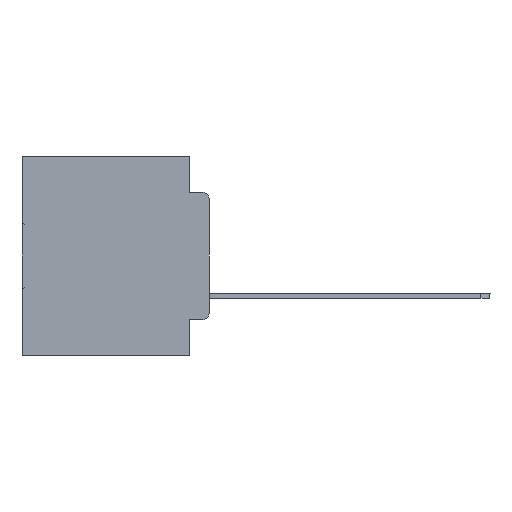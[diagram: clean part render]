
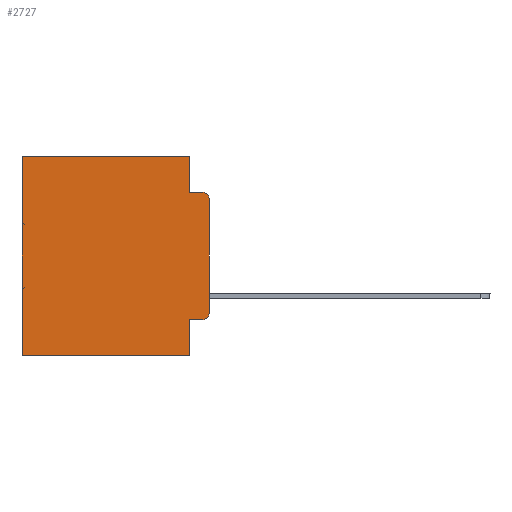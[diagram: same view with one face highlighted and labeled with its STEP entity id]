
A CAD part, left-side view. The second image highlights one B-rep face of the part: STEP entity #2727.
In plain terms, the highlighted planar face has unit normal (-1, 0, 0).
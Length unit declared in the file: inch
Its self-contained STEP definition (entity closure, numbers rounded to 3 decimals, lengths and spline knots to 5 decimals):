
#1617 = DIRECTION ( 'NONE',  ( 0., -1., 0. ) ) ;
#2645 = LINE ( 'NONE', #10070, #27290 ) ;
#2679 = ORIENTED_EDGE ( 'NONE', *, *, #4344, .F. ) ;
#2701 = ORIENTED_EDGE ( 'NONE', *, *, #13896, .F. ) ;
#2727 = ADVANCED_FACE ( 'NONE', ( #23190 ), #23687, .F. ) ;
#3690 = CARTESIAN_POINT ( 'NONE',  ( 0.298, 0.02, -0.4115 ) ) ;
#4344 = EDGE_CURVE ( 'NONE', #23893, #30418, #20851, .T. ) ;
#5278 = VERTEX_POINT ( 'NONE', #13805 ) ;
#5730 = DIRECTION ( 'NONE',  ( 0., 0., -1. ) ) ;
#6343 = ORIENTED_EDGE ( 'NONE', *, *, #31186, .F. ) ;
#6917 = LINE ( 'NONE', #28283, #15752 ) ;
#7305 = DIRECTION ( 'NONE',  ( 0., 0., -1. ) ) ;
#7715 = DIRECTION ( 'NONE',  ( 0., 0., -1. ) ) ;
#8088 = CARTESIAN_POINT ( 'NONE',  ( 0.298, 0.051, 0. ) ) ;
#8089 = DIRECTION ( 'NONE',  ( 1., 0., 0. ) ) ;
#8579 = CARTESIAN_POINT ( 'NONE',  ( 0.298, 0., -0.5 ) ) ;
#9032 = VERTEX_POINT ( 'NONE', #23103 ) ;
#9220 = VERTEX_POINT ( 'NONE', #29182 ) ;
#9267 = ORIENTED_EDGE ( 'NONE', *, *, #15329, .T. ) ;
#9557 = VERTEX_POINT ( 'NONE', #3690 ) ;
#9857 = EDGE_CURVE ( 'NONE', #23893, #5278, #28074, .T. ) ;
#10055 = LINE ( 'NONE', #28208, #25233 ) ;
#10070 = CARTESIAN_POINT ( 'NONE',  ( 0.298, 0., 0. ) ) ;
#11087 = CARTESIAN_POINT ( 'NONE',  ( 0.298, 0.473, -0.5 ) ) ;
#11134 = VECTOR ( 'NONE', #24522, 39.37008 ) ;
#11430 = AXIS2_PLACEMENT_3D ( 'NONE', #30977, #8089, #5730 ) ;
#11694 = ORIENTED_EDGE ( 'NONE', *, *, #18281, .T. ) ;
#12052 = DIRECTION ( 'NONE',  ( 0., 0., -1. ) ) ;
#12464 = CARTESIAN_POINT ( 'NONE',  ( 0.298, 0.02, -0.1085 ) ) ;
#12587 = VERTEX_POINT ( 'NONE', #25571 ) ;
#12720 = DIRECTION ( 'NONE',  ( 0., 0., -1. ) ) ;
#12936 = DIRECTION ( 'NONE',  ( 0., -1., 0. ) ) ;
#12950 = DIRECTION ( 'NONE',  ( 0., 1., 0. ) ) ;
#13708 = VECTOR ( 'NONE', #12720, 39.37008 ) ;
#13805 = CARTESIAN_POINT ( 'NONE',  ( 0.298, 0.02, -0.0885 ) ) ;
#13896 = EDGE_CURVE ( 'NONE', #14059, #12587, #6917, .T. ) ;
#13926 = CARTESIAN_POINT ( 'NONE',  ( 0.298, 0.051, 0. ) ) ;
#14059 = VERTEX_POINT ( 'NONE', #8088 ) ;
#14183 = CIRCLE ( 'NONE', #32062, 0.02 ) ;
#15329 = EDGE_CURVE ( 'NONE', #9557, #30418, #14183, .T. ) ;
#15752 = VECTOR ( 'NONE', #19982, 39.37008 ) ;
#16455 = VECTOR ( 'NONE', #1617, 39.37008 ) ;
#17025 = LINE ( 'NONE', #19911, #16455 ) ;
#17555 = DIRECTION ( 'NONE',  ( -1., 0., 0. ) ) ;
#18143 = DIRECTION ( 'NONE',  ( -1., 0., 0. ) ) ;
#18281 = EDGE_CURVE ( 'NONE', #14059, #23511, #2645, .T. ) ;
#19208 = EDGE_LOOP ( 'NONE', ( #2679, #32222, #6343, #2701, #11694, #20461, #23949, #25158, #27980, #9267 ) ) ;
#19210 = DIRECTION ( 'NONE',  ( 0., 0., -1. ) ) ;
#19722 = CARTESIAN_POINT ( 'NONE',  ( 0.298, 0.473, 0. ) ) ;
#19911 = CARTESIAN_POINT ( 'NONE',  ( 0.298, 0.051, -0.4115 ) ) ;
#19953 = VERTEX_POINT ( 'NONE', #11087 ) ;
#19982 = DIRECTION ( 'NONE',  ( 0., 0., -1. ) ) ;
#20213 = EDGE_CURVE ( 'NONE', #23511, #19953, #24472, .T. ) ;
#20461 = ORIENTED_EDGE ( 'NONE', *, *, #20213, .T. ) ;
#20851 = LINE ( 'NONE', #26293, #13708 ) ;
#23061 = VECTOR ( 'NONE', #19210, 39.37008 ) ;
#23103 = CARTESIAN_POINT ( 'NONE',  ( 0.298, 0.051, -0.5 ) ) ;
#23188 = EDGE_CURVE ( 'NONE', #9220, #9032, #24946, .T. ) ;
#23190 = FACE_OUTER_BOUND ( 'NONE', #19208, .T. ) ;
#23511 = VERTEX_POINT ( 'NONE', #25464 ) ;
#23687 = PLANE ( 'NONE',  #11430 ) ;
#23893 = VERTEX_POINT ( 'NONE', #24403 ) ;
#23949 = ORIENTED_EDGE ( 'NONE', *, *, #30480, .F. ) ;
#24018 = LINE ( 'NONE', #8579, #11134 ) ;
#24403 = CARTESIAN_POINT ( 'NONE',  ( 0.298, 0., -0.1085 ) ) ;
#24472 = LINE ( 'NONE', #19722, #23061 ) ;
#24522 = DIRECTION ( 'NONE',  ( 0., 1., 0. ) ) ;
#24946 = LINE ( 'NONE', #13926, #28575 ) ;
#25158 = ORIENTED_EDGE ( 'NONE', *, *, #23188, .F. ) ;
#25233 = VECTOR ( 'NONE', #12936, 39.37008 ) ;
#25464 = CARTESIAN_POINT ( 'NONE',  ( 0.298, 0.473, 0. ) ) ;
#25571 = CARTESIAN_POINT ( 'NONE',  ( 0.298, 0.051, -0.0885 ) ) ;
#26293 = CARTESIAN_POINT ( 'NONE',  ( 0.298, 0., 0. ) ) ;
#27290 = VECTOR ( 'NONE', #12950, 39.37008 ) ;
#27345 = EDGE_CURVE ( 'NONE', #9220, #9557, #17025, .T. ) ;
#27980 = ORIENTED_EDGE ( 'NONE', *, *, #27345, .T. ) ;
#28074 = CIRCLE ( 'NONE', #32382, 0.02 ) ;
#28208 = CARTESIAN_POINT ( 'NONE',  ( 0.298, 0.051, -0.0885 ) ) ;
#28283 = CARTESIAN_POINT ( 'NONE',  ( 0.298, 0.051, 0. ) ) ;
#28329 = CARTESIAN_POINT ( 'NONE',  ( 0.298, 0.02, -0.3915 ) ) ;
#28575 = VECTOR ( 'NONE', #12052, 39.37008 ) ;
#29182 = CARTESIAN_POINT ( 'NONE',  ( 0.298, 0.051, -0.4115 ) ) ;
#29269 = CARTESIAN_POINT ( 'NONE',  ( 0.298, 0., -0.3915 ) ) ;
#30418 = VERTEX_POINT ( 'NONE', #29269 ) ;
#30480 = EDGE_CURVE ( 'NONE', #9032, #19953, #24018, .T. ) ;
#30977 = CARTESIAN_POINT ( 'NONE',  ( 0.298, 0., 0. ) ) ;
#31186 = EDGE_CURVE ( 'NONE', #12587, #5278, #10055, .T. ) ;
#32062 = AXIS2_PLACEMENT_3D ( 'NONE', #28329, #18143, #7305 ) ;
#32222 = ORIENTED_EDGE ( 'NONE', *, *, #9857, .T. ) ;
#32382 = AXIS2_PLACEMENT_3D ( 'NONE', #12464, #17555, #7715 ) ;
